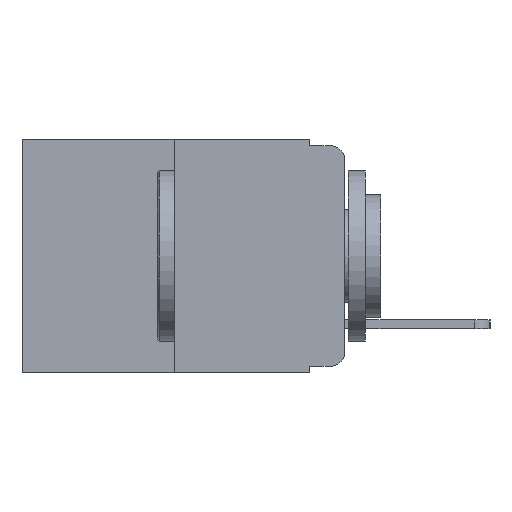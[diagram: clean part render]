
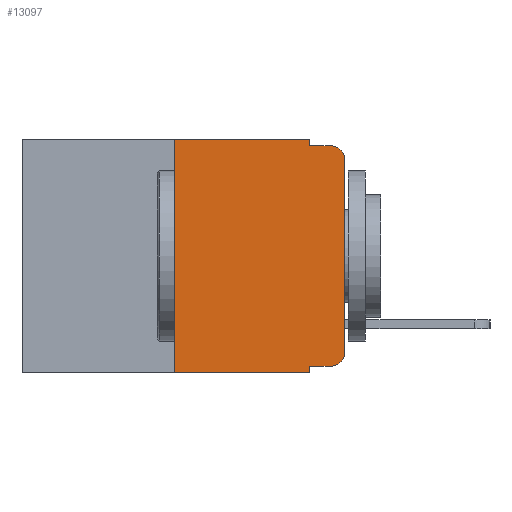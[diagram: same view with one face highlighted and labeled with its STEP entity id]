
A CAD part, left-side view. The second image highlights one B-rep face of the part: STEP entity #13097.
In plain terms, the highlighted planar face has unit normal (-1, 0, 0).
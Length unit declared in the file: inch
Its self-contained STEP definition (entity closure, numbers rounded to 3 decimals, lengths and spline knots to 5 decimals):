
#805 = EDGE_LOOP ( 'NONE', ( #8379, #18983, #19610, #4328, #2121, #18036, #8082, #18685, #24560, #25787 ) ) ;
#1220 = DIRECTION ( 'NONE',  ( 0., 0., -1. ) ) ;
#1444 = VECTOR ( 'NONE', #19418, 39.37008 ) ;
#1634 = CARTESIAN_POINT ( 'NONE',  ( 0., 0.051, 0. ) ) ;
#1651 = CARTESIAN_POINT ( 'NONE',  ( 0., 0., 0. ) ) ;
#1661 = CARTESIAN_POINT ( 'NONE',  ( 0., 0.051, 0. ) ) ;
#2059 = VERTEX_POINT ( 'NONE', #1634 ) ;
#2092 = LINE ( 'NONE', #7481, #1444 ) ;
#2121 = ORIENTED_EDGE ( 'NONE', *, *, #13792, .F. ) ;
#2177 = CARTESIAN_POINT ( 'NONE',  ( 0., 0., -0.03 ) ) ;
#2412 = EDGE_CURVE ( 'NONE', #9837, #10233, #18684, .T. ) ;
#2969 = CARTESIAN_POINT ( 'NONE',  ( 0., 0.02, -0.01 ) ) ;
#3120 = FACE_OUTER_BOUND ( 'NONE', #805, .T. ) ;
#3191 = CIRCLE ( 'NONE', #5043, 0.02 ) ;
#3193 = CIRCLE ( 'NONE', #8048, 0.02 ) ;
#3966 = VECTOR ( 'NONE', #10544, 39.37008 ) ;
#4328 = ORIENTED_EDGE ( 'NONE', *, *, #6437, .F. ) ;
#4546 = VERTEX_POINT ( 'NONE', #2177 ) ;
#4548 = CARTESIAN_POINT ( 'NONE',  ( 0., 0.051, -0.343 ) ) ;
#4940 = VERTEX_POINT ( 'NONE', #9498 ) ;
#5043 = AXIS2_PLACEMENT_3D ( 'NONE', #25098, #13195, #1220 ) ;
#5076 = EDGE_CURVE ( 'NONE', #22354, #16810, #7655, .T. ) ;
#5330 = VERTEX_POINT ( 'NONE', #22547 ) ;
#5553 = AXIS2_PLACEMENT_3D ( 'NONE', #5616, #23543, #11634 ) ;
#5616 = CARTESIAN_POINT ( 'NONE',  ( 0., 0.473, 0. ) ) ;
#5940 = CARTESIAN_POINT ( 'NONE',  ( 0., 0., -0.313 ) ) ;
#5955 = CARTESIAN_POINT ( 'NONE',  ( 0., 0.25, 0. ) ) ;
#6437 = EDGE_CURVE ( 'NONE', #2059, #5330, #8876, .T. ) ;
#6584 = CARTESIAN_POINT ( 'NONE',  ( 0., 0.473, -0.343 ) ) ;
#7464 = VECTOR ( 'NONE', #17852, 39.37008 ) ;
#7481 = CARTESIAN_POINT ( 'NONE',  ( 0., 0.051, -0.333 ) ) ;
#7630 = PLANE ( 'NONE',  #5553 ) ;
#7655 = LINE ( 'NONE', #17835, #17607 ) ;
#7773 = EDGE_CURVE ( 'NONE', #5330, #25356, #12854, .T. ) ;
#7958 = CARTESIAN_POINT ( 'NONE',  ( 0., 0.02, -0.03 ) ) ;
#8048 = AXIS2_PLACEMENT_3D ( 'NONE', #7958, #21904, #9963 ) ;
#8082 = ORIENTED_EDGE ( 'NONE', *, *, #24591, .T. ) ;
#8379 = ORIENTED_EDGE ( 'NONE', *, *, #13110, .T. ) ;
#8876 = LINE ( 'NONE', #1661, #24121 ) ;
#9498 = CARTESIAN_POINT ( 'NONE',  ( 0., 0.02, -0.333 ) ) ;
#9837 = VERTEX_POINT ( 'NONE', #15368 ) ;
#9963 = DIRECTION ( 'NONE',  ( 0., 0., -1. ) ) ;
#10233 = VERTEX_POINT ( 'NONE', #4548 ) ;
#10544 = DIRECTION ( 'NONE',  ( 0., -1., 0. ) ) ;
#11173 = CARTESIAN_POINT ( 'NONE',  ( 0., 0.25, -0.343 ) ) ;
#11634 = DIRECTION ( 'NONE',  ( 0., 0., -1. ) ) ;
#11780 = EDGE_CURVE ( 'NONE', #4546, #25356, #3193, .T. ) ;
#12490 = LINE ( 'NONE', #1651, #22467 ) ;
#12854 = LINE ( 'NONE', #21864, #17507 ) ;
#13097 = ADVANCED_FACE ( 'NONE', ( #3120 ), #7630, .F. ) ;
#13110 = EDGE_CURVE ( 'NONE', #19342, #4546, #12490, .T. ) ;
#13195 = DIRECTION ( 'NONE',  ( -1., 0., 0. ) ) ;
#13792 = EDGE_CURVE ( 'NONE', #16810, #2059, #23339, .T. ) ;
#15368 = CARTESIAN_POINT ( 'NONE',  ( 0., 0.051, -0.333 ) ) ;
#15868 = CARTESIAN_POINT ( 'NONE',  ( 0., 0.473, 0. ) ) ;
#16810 = VERTEX_POINT ( 'NONE', #5955 ) ;
#17507 = VECTOR ( 'NONE', #25811, 39.37008 ) ;
#17607 = VECTOR ( 'NONE', #21867, 39.37008 ) ;
#17835 = CARTESIAN_POINT ( 'NONE',  ( 0., 0.25, 0. ) ) ;
#17852 = DIRECTION ( 'NONE',  ( 0., -1., 0. ) ) ;
#18036 = ORIENTED_EDGE ( 'NONE', *, *, #5076, .F. ) ;
#18431 = CARTESIAN_POINT ( 'NONE',  ( 0., 0.051, 0. ) ) ;
#18587 = DIRECTION ( 'NONE',  ( 0., 0., -1. ) ) ;
#18684 = LINE ( 'NONE', #18431, #24559 ) ;
#18685 = ORIENTED_EDGE ( 'NONE', *, *, #2412, .F. ) ;
#18983 = ORIENTED_EDGE ( 'NONE', *, *, #11780, .T. ) ;
#19342 = VERTEX_POINT ( 'NONE', #5940 ) ;
#19418 = DIRECTION ( 'NONE',  ( 0., -1., 0. ) ) ;
#19610 = ORIENTED_EDGE ( 'NONE', *, *, #7773, .F. ) ;
#19663 = DIRECTION ( 'NONE',  ( 0., 0., 1. ) ) ;
#21864 = CARTESIAN_POINT ( 'NONE',  ( 0., 0.051, -0.01 ) ) ;
#21867 = DIRECTION ( 'NONE',  ( 0., 0., 1. ) ) ;
#21904 = DIRECTION ( 'NONE',  ( -1., 0., 0. ) ) ;
#22354 = VERTEX_POINT ( 'NONE', #11173 ) ;
#22467 = VECTOR ( 'NONE', #19663, 39.37008 ) ;
#22547 = CARTESIAN_POINT ( 'NONE',  ( 0., 0.051, -0.01 ) ) ;
#22963 = EDGE_CURVE ( 'NONE', #4940, #19342, #3191, .T. ) ;
#23339 = LINE ( 'NONE', #15868, #7464 ) ;
#23543 = DIRECTION ( 'NONE',  ( 1., 0., 0. ) ) ;
#24121 = VECTOR ( 'NONE', #25532, 39.37008 ) ;
#24261 = EDGE_CURVE ( 'NONE', #9837, #4940, #2092, .T. ) ;
#24559 = VECTOR ( 'NONE', #18587, 39.37008 ) ;
#24560 = ORIENTED_EDGE ( 'NONE', *, *, #24261, .T. ) ;
#24591 = EDGE_CURVE ( 'NONE', #22354, #10233, #25122, .T. ) ;
#25098 = CARTESIAN_POINT ( 'NONE',  ( 0., 0.02, -0.313 ) ) ;
#25122 = LINE ( 'NONE', #6584, #3966 ) ;
#25356 = VERTEX_POINT ( 'NONE', #2969 ) ;
#25532 = DIRECTION ( 'NONE',  ( 0., 0., -1. ) ) ;
#25787 = ORIENTED_EDGE ( 'NONE', *, *, #22963, .T. ) ;
#25811 = DIRECTION ( 'NONE',  ( 0., -1., 0. ) ) ;
